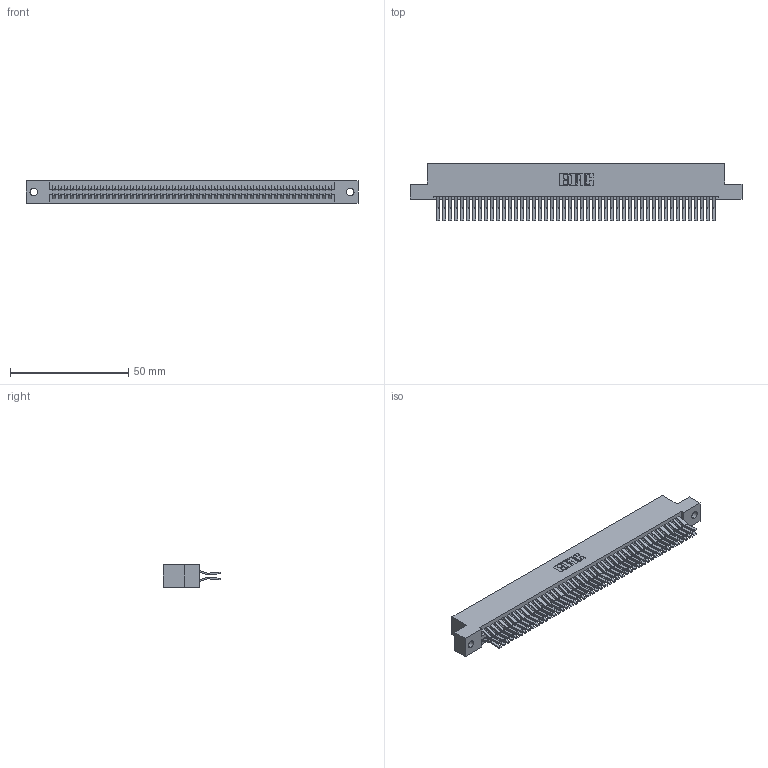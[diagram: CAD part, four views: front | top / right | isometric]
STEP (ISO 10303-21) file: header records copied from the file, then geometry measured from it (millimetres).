
FILE_DESCRIPTION (( 'STEP AP203' ), '1' );
FILE_NAME ('395-094-560-202.STEP', '2019-10-25T23:26:24', ( '' ), ( '' ), 'SwSTEP 2.0', 'SolidWorks 2016', '' );
FILE_SCHEMA (( 'CONFIG_CONTROL_DESIGN' ));
Length unit declared in the file: inch
Products named in the file (3): 345-292-001_560 Tail; 395-094-560-202; 345 Part_Flush Mounting Lugs - 0.128 Dia
Assembly tree (95 placements, depth 2):
  395-094-560-202
    345 Part_Flush Mounting Lugs - 0.128 Dia
    345-292-001_560 Tail  x94
Bounding box: 140.59 x 24.45 x 9.4 mm (x, y, z)
Volume: 14282.8 mm3; surface area: 22521.2 mm2
Topology: 95 solids, 95 shells, 5014 faces, 14911 edges, 9814 vertices
Faces by surface type: plane 3182, cylinder 1832
Entity records: 36295 total; most frequent: CARTESIAN_POINT 6080, ORIENTED_EDGE 6014, DIRECTION 5359, EDGE_CURVE 3007, VECTOR 2683, LINE 2683, VERTEX_POINT 2002, AXIS2_PLACEMENT_3D 1338
